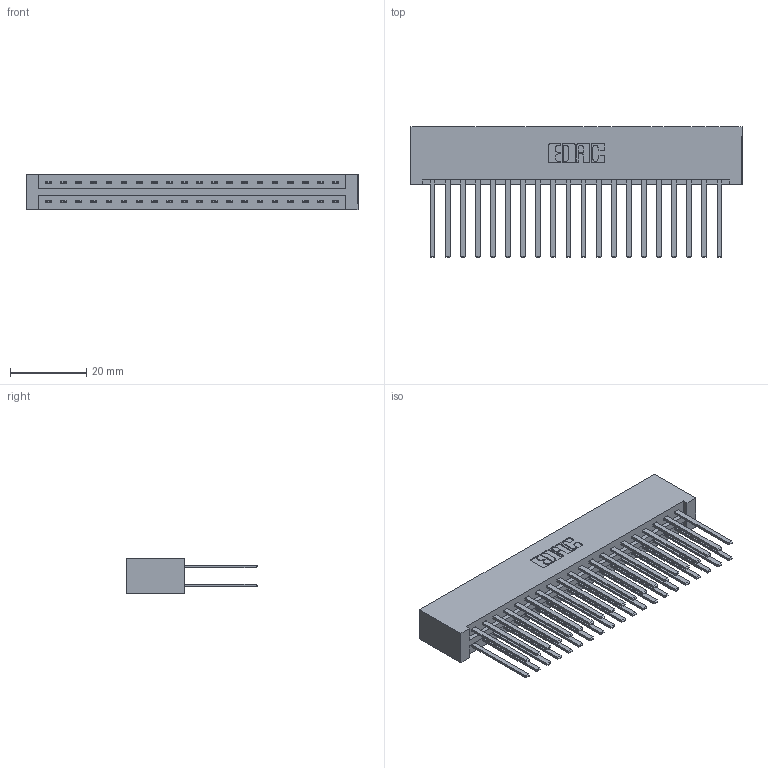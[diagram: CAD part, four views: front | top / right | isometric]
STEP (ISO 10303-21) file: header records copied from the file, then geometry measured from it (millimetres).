
FILE_DESCRIPTION (( 'STEP AP203' ), '1' );
FILE_NAME ('387-040-544-201.STEP', '2019-10-18T02:55:43', ( '' ), ( '' ), 'SwSTEP 2.0', 'SolidWorks 2016', '' );
FILE_SCHEMA (( 'CONFIG_CONTROL_DESIGN' ));
Length unit declared in the file: inch
Products named in the file (3): 387-040-544-201; 345-292-001_345-293-144; 337 Part_No Mounting Lugs
Assembly tree (41 placements, depth 2):
  387-040-544-201
    337 Part_No Mounting Lugs
    345-292-001_345-293-144  x40
Bounding box: 87.12 x 34.3 x 9.4 mm (x, y, z)
Volume: 10210.2 mm3; surface area: 13216.8 mm2
Topology: 41 solids, 41 shells, 2026 faces, 6007 edges, 3950 vertices
Faces by surface type: plane 1426, cylinder 600
Entity records: 17891 total; most frequent: CARTESIAN_POINT 3030, ORIENTED_EDGE 2966, DIRECTION 2607, EDGE_CURVE 1483, VECTOR 1367, LINE 1367, VERTEX_POINT 986, AXIS2_PLACEMENT_3D 620
